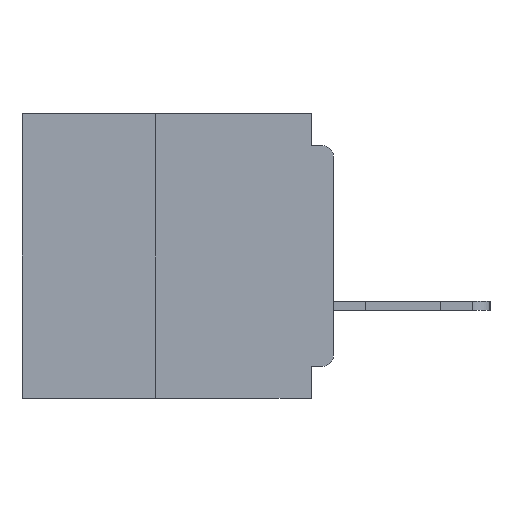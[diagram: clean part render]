
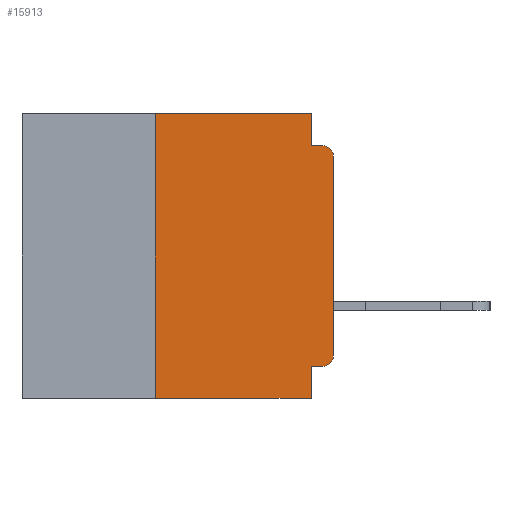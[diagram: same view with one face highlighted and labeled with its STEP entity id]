
A CAD part, left-side view. The second image highlights one B-rep face of the part: STEP entity #15913.
In plain terms, the highlighted planar face has unit normal (-1, 0, 0).
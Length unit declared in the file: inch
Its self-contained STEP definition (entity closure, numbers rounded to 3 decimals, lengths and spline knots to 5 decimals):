
#181 = DIRECTION ( 'NONE',  ( 0., -1., 0. ) ) ;
#318 = VECTOR ( 'NONE', #11011, 39.37008 ) ;
#375 = CARTESIAN_POINT ( 'NONE',  ( 0., 0., 0. ) ) ;
#937 = AXIS2_PLACEMENT_3D ( 'NONE', #16974, #46636, #21223 ) ;
#1821 = CARTESIAN_POINT ( 'NONE',  ( 0., 0., -0.34 ) ) ;
#3324 = LINE ( 'NONE', #14777, #37298 ) ;
#3904 = FACE_OUTER_BOUND ( 'NONE', #22643, .T. ) ;
#4364 = DIRECTION ( 'NONE',  ( 0., -1., 0. ) ) ;
#4534 = VECTOR ( 'NONE', #20735, 39.37008 ) ;
#4676 = CIRCLE ( 'NONE', #937, 0.015 ) ;
#6725 = VECTOR ( 'NONE', #36670, 39.37008 ) ;
#6798 = LINE ( 'NONE', #17114, #49151 ) ;
#7246 = ORIENTED_EDGE ( 'NONE', *, *, #49197, .F. ) ;
#7261 = ORIENTED_EDGE ( 'NONE', *, *, #23041, .F. ) ;
#8987 = CARTESIAN_POINT ( 'NONE',  ( 0., 0.015, -0.355 ) ) ;
#9417 = VERTEX_POINT ( 'NONE', #16826 ) ;
#10334 = EDGE_CURVE ( 'NONE', #42681, #45010, #17973, .T. ) ;
#11011 = DIRECTION ( 'NONE',  ( 0., 1., 0. ) ) ;
#11979 = VERTEX_POINT ( 'NONE', #47300 ) ;
#14777 = CARTESIAN_POINT ( 'NONE',  ( 0., 0.031, 0. ) ) ;
#14840 = CARTESIAN_POINT ( 'NONE',  ( 0., 0.015, -0.06 ) ) ;
#15015 = CARTESIAN_POINT ( 'NONE',  ( 0., 0.031, -0.4 ) ) ;
#15578 = ORIENTED_EDGE ( 'NONE', *, *, #51337, .T. ) ;
#15913 = ADVANCED_FACE ( 'NONE', ( #3904 ), #21204, .F. ) ;
#16500 = CARTESIAN_POINT ( 'NONE',  ( 0., 0.25, -0.4 ) ) ;
#16790 = ORIENTED_EDGE ( 'NONE', *, *, #29832, .T. ) ;
#16826 = CARTESIAN_POINT ( 'NONE',  ( 0., 0.015, -0.045 ) ) ;
#16974 = CARTESIAN_POINT ( 'NONE',  ( 0., 0.015, -0.34 ) ) ;
#16987 = CARTESIAN_POINT ( 'NONE',  ( 0., 0., -0.045 ) ) ;
#17114 = CARTESIAN_POINT ( 'NONE',  ( 0., 0.437, -0.4 ) ) ;
#17130 = DIRECTION ( 'NONE',  ( 0., 0., -1. ) ) ;
#17708 = VERTEX_POINT ( 'NONE', #8987 ) ;
#17973 = LINE ( 'NONE', #32373, #6725 ) ;
#18395 = VECTOR ( 'NONE', #51296, 39.37008 ) ;
#18996 = DIRECTION ( 'NONE',  ( 0., 0., -1. ) ) ;
#19067 = DIRECTION ( 'NONE',  ( 0., 0., -1. ) ) ;
#20735 = DIRECTION ( 'NONE',  ( 0., 0., 1. ) ) ;
#21204 = PLANE ( 'NONE',  #50134 ) ;
#21223 = DIRECTION ( 'NONE',  ( 0., 0., -1. ) ) ;
#22643 = EDGE_LOOP ( 'NONE', ( #15578, #28066, #7261, #7246, #44595, #34674, #44039, #44532, #27709, #16790 ) ) ;
#22721 = CARTESIAN_POINT ( 'NONE',  ( 0., 0.031, -0.045 ) ) ;
#23041 = EDGE_CURVE ( 'NONE', #38990, #9417, #52800, .T. ) ;
#27252 = AXIS2_PLACEMENT_3D ( 'NONE', #14840, #44521, #19067 ) ;
#27709 = ORIENTED_EDGE ( 'NONE', *, *, #52365, .F. ) ;
#28066 = ORIENTED_EDGE ( 'NONE', *, *, #38412, .T. ) ;
#28225 = VERTEX_POINT ( 'NONE', #45828 ) ;
#29750 = LINE ( 'NONE', #375, #18395 ) ;
#29832 = EDGE_CURVE ( 'NONE', #17708, #35009, #4676, .T. ) ;
#32306 = EDGE_CURVE ( 'NONE', #11979, #50487, #46213, .T. ) ;
#32373 = CARTESIAN_POINT ( 'NONE',  ( 0., 0.437, 0. ) ) ;
#33683 = VECTOR ( 'NONE', #48317, 39.37008 ) ;
#34674 = ORIENTED_EDGE ( 'NONE', *, *, #43646, .F. ) ;
#35009 = VERTEX_POINT ( 'NONE', #1821 ) ;
#35138 = CARTESIAN_POINT ( 'NONE',  ( 0., 0.031, 0. ) ) ;
#36670 = DIRECTION ( 'NONE',  ( 0., -1., 0. ) ) ;
#37298 = VECTOR ( 'NONE', #18996, 39.37008 ) ;
#38366 = CARTESIAN_POINT ( 'NONE',  ( 0., 0.437, 0. ) ) ;
#38412 = EDGE_CURVE ( 'NONE', #28225, #9417, #51942, .T. ) ;
#38476 = LINE ( 'NONE', #16500, #4534 ) ;
#38990 = VERTEX_POINT ( 'NONE', #22721 ) ;
#40833 = EDGE_CURVE ( 'NONE', #43550, #50487, #6798, .T. ) ;
#41794 = VECTOR ( 'NONE', #4364, 39.37008 ) ;
#42619 = DIRECTION ( 'NONE',  ( 1., 0., 0. ) ) ;
#42681 = VERTEX_POINT ( 'NONE', #46752 ) ;
#43550 = VERTEX_POINT ( 'NONE', #49396 ) ;
#43646 = EDGE_CURVE ( 'NONE', #43550, #42681, #38476, .T. ) ;
#44039 = ORIENTED_EDGE ( 'NONE', *, *, #40833, .T. ) ;
#44521 = DIRECTION ( 'NONE',  ( -1., 0., 0. ) ) ;
#44532 = ORIENTED_EDGE ( 'NONE', *, *, #32306, .F. ) ;
#44595 = ORIENTED_EDGE ( 'NONE', *, *, #10334, .F. ) ;
#45010 = VERTEX_POINT ( 'NONE', #35138 ) ;
#45828 = CARTESIAN_POINT ( 'NONE',  ( 0., 0., -0.06 ) ) ;
#46213 = LINE ( 'NONE', #48496, #33683 ) ;
#46636 = DIRECTION ( 'NONE',  ( -1., 0., 0. ) ) ;
#46752 = CARTESIAN_POINT ( 'NONE',  ( 0., 0.25, 0. ) ) ;
#47300 = CARTESIAN_POINT ( 'NONE',  ( 0., 0.031, -0.355 ) ) ;
#48317 = DIRECTION ( 'NONE',  ( 0., 0., -1. ) ) ;
#48496 = CARTESIAN_POINT ( 'NONE',  ( 0., 0.031, -0.4 ) ) ;
#49151 = VECTOR ( 'NONE', #181, 39.37008 ) ;
#49197 = EDGE_CURVE ( 'NONE', #45010, #38990, #3324, .T. ) ;
#49396 = CARTESIAN_POINT ( 'NONE',  ( 0., 0.25, -0.4 ) ) ;
#50134 = AXIS2_PLACEMENT_3D ( 'NONE', #38366, #42619, #17130 ) ;
#50487 = VERTEX_POINT ( 'NONE', #15015 ) ;
#51296 = DIRECTION ( 'NONE',  ( 0., 0., 1. ) ) ;
#51337 = EDGE_CURVE ( 'NONE', #35009, #28225, #29750, .T. ) ;
#51942 = CIRCLE ( 'NONE', #27252, 0.015 ) ;
#52365 = EDGE_CURVE ( 'NONE', #17708, #11979, #53961, .T. ) ;
#52800 = LINE ( 'NONE', #16987, #41794 ) ;
#53265 = CARTESIAN_POINT ( 'NONE',  ( 0., 0., -0.355 ) ) ;
#53961 = LINE ( 'NONE', #53265, #318 ) ;
